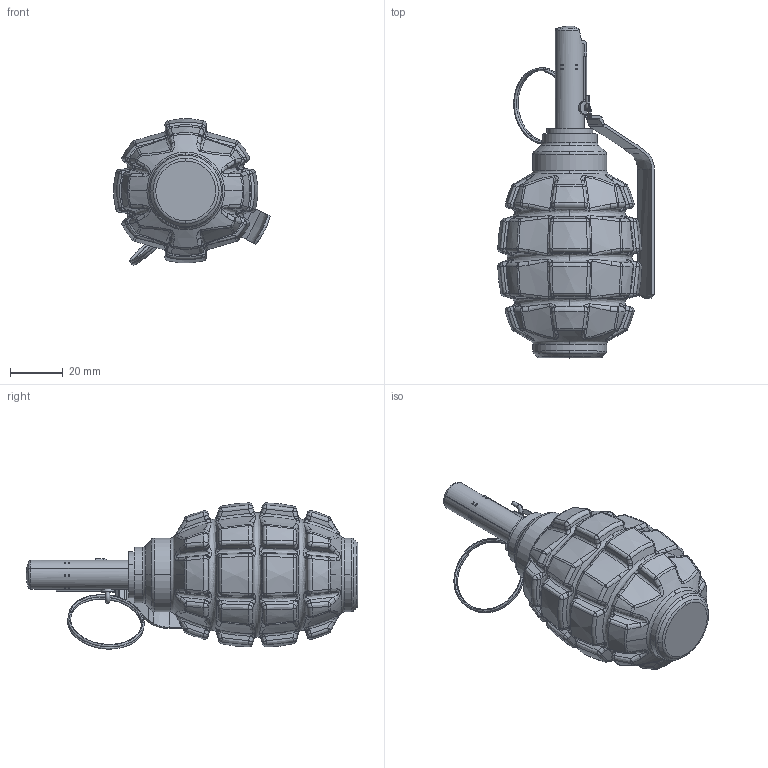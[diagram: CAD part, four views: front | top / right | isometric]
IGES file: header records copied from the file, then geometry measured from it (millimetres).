
Global section: file name: HNo Iges File Name specified; native system: Autodesk Inventor 2011; preprocessor: AutoDesk Inventor Iges Exporter R2011; author: EfimchenkoPA; date: 20111028.092332; units: millimetre
Bounding box: 59.41 x 126 x 55.48 mm (x, y, z)
Volume: 116618.5 mm3; surface area: 28076.6 mm2
Topology: 10 solids, 10 shells, 1176 faces, 2758 edges, 1622 vertices
Faces by surface type: bspline 485, plane 201, sphere 130, revolution 99, cone 97, torus 90, cylinder 74
